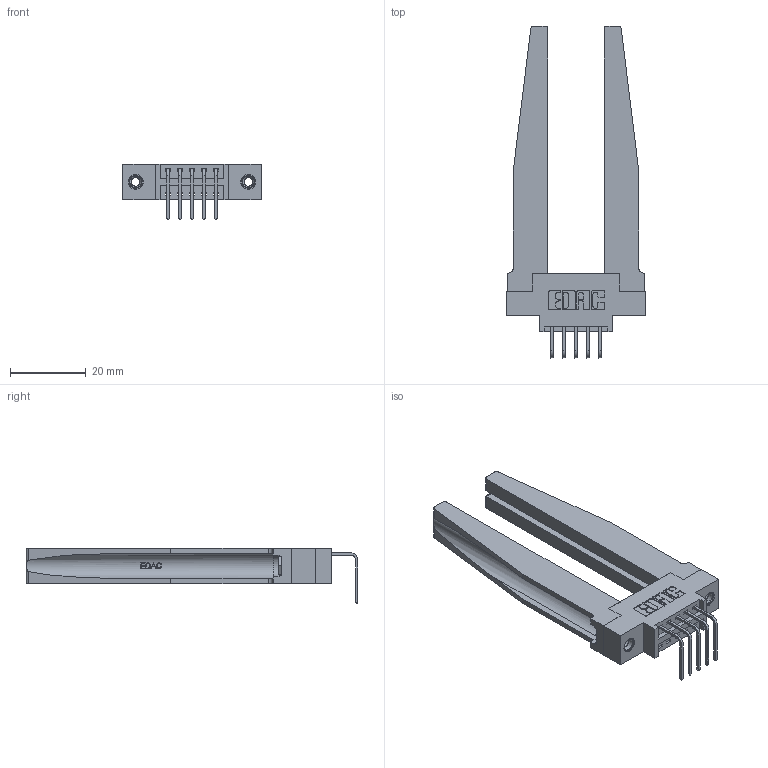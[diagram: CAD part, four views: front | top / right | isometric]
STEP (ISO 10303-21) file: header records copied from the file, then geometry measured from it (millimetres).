
FILE_DESCRIPTION (( 'STEP AP203' ), '1' );
FILE_NAME ('396-005-558-678.STEP', '2022-05-17T07:15:24', ( '' ), ( '' ), 'SwSTEP 2.0', 'SolidWorks 2020', '' );
FILE_SCHEMA (( 'CONFIG_CONTROL_DESIGN' ));
Length unit declared in the file: inch
Products named in the file (5): 396-005-558-678; 346 Part_0.170 Offset - 0.156 Dia-TH; 345-292-001_558 Tail - 2; 345-250-001_345-250-001-102; 346-220-078_345-220-078
Assembly tree (10 placements, depth 2):
  396-005-558-678
    346 Part_0.170 Offset - 0.156 Dia-TH
    345-292-001_558 Tail - 2  x5
    346-220-078_345-220-078  x2
    345-250-001_345-250-001-102  x2
Bounding box: 36.45 x 87.44 x 14.73 mm (x, y, z)
Volume: 9986.9 mm3; surface area: 10279.9 mm2
Topology: 10 solids, 10 shells, 674 faces, 1895 edges, 1246 vertices
Faces by surface type: plane 446, cylinder 176, bspline 36, cone 12, torus 4
Entity records: 13464 total; most frequent: CARTESIAN_POINT 3236, ORIENTED_EDGE 2062, DIRECTION 1883, EDGE_CURVE 1031, VECTOR 785, LINE 785, VERTEX_POINT 680, AXIS2_PLACEMENT_3D 549
